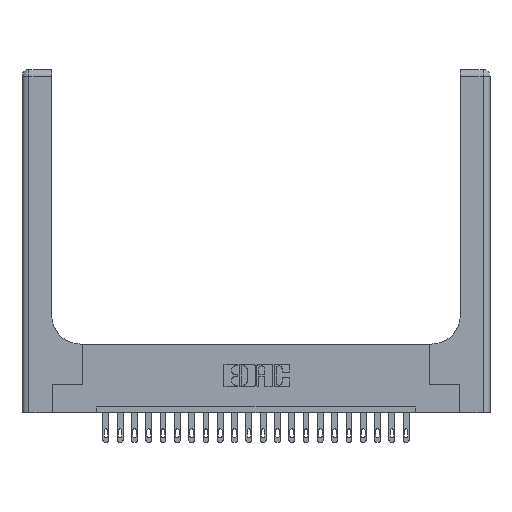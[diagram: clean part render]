
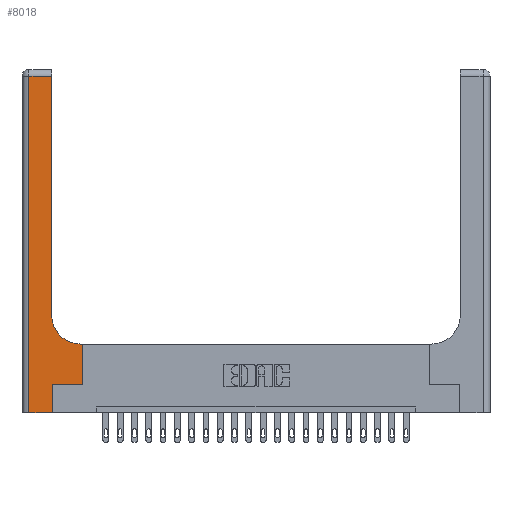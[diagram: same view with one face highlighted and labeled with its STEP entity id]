
A CAD part, top view. The second image highlights one B-rep face of the part: STEP entity #8018.
In plain terms, the highlighted planar face has unit normal (0, 0, 1).
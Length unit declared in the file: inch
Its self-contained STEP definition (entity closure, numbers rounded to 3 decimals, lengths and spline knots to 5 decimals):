
#81 = CARTESIAN_POINT ( 'NONE',  ( 0.528, 0.25, 0.37 ) ) ;
#326 = CARTESIAN_POINT ( 'NONE',  ( 0.26, 2.94, 0.37 ) ) ;
#426 = CARTESIAN_POINT ( 'NONE',  ( 0., 0., 0.37 ) ) ;
#790 = DIRECTION ( 'NONE',  ( 1., 0., 0. ) ) ;
#1011 = CARTESIAN_POINT ( 'NONE',  ( 0.265, 0., 0.37 ) ) ;
#1046 = DIRECTION ( 'NONE',  ( -1., 0., 0. ) ) ;
#1199 = DIRECTION ( 'NONE',  ( -1., 0., 0. ) ) ;
#1802 = CARTESIAN_POINT ( 'NONE',  ( 0.265, 0., 0.37 ) ) ;
#2324 = VERTEX_POINT ( 'NONE', #20525 ) ;
#2341 = CARTESIAN_POINT ( 'NONE',  ( 0.51, 0.85, 0.37 ) ) ;
#2616 = DIRECTION ( 'NONE',  ( 1., 0., 0. ) ) ;
#2735 = CIRCLE ( 'NONE', #18642, 0.25 ) ;
#2833 = VERTEX_POINT ( 'NONE', #18940 ) ;
#3242 = DIRECTION ( 'NONE',  ( 0., 1., 0. ) ) ;
#3520 = LINE ( 'NONE', #81, #6730 ) ;
#3695 = LINE ( 'NONE', #1802, #6019 ) ;
#4494 = CARTESIAN_POINT ( 'NONE',  ( 0., 2.94, 0.37 ) ) ;
#4508 = VECTOR ( 'NONE', #1046, 39.37008 ) ;
#5003 = EDGE_CURVE ( 'NONE', #10012, #18430, #2735, .T. ) ;
#5129 = ORIENTED_EDGE ( 'NONE', *, *, #12434, .T. ) ;
#5174 = DIRECTION ( 'NONE',  ( 0., 1., 0. ) ) ;
#5262 = VECTOR ( 'NONE', #20151, 39.37008 ) ;
#5644 = VERTEX_POINT ( 'NONE', #13246 ) ;
#5827 = DIRECTION ( 'NONE',  ( -1., 0., 0. ) ) ;
#5969 = EDGE_CURVE ( 'NONE', #21880, #2833, #12785, .T. ) ;
#6019 = VECTOR ( 'NONE', #3242, 39.37008 ) ;
#6056 = EDGE_CURVE ( 'NONE', #21258, #5644, #11017, .T. ) ;
#6388 = CARTESIAN_POINT ( 'NONE',  ( 0., 3., 0.37 ) ) ;
#6585 = CARTESIAN_POINT ( 'NONE',  ( 0.26, 0.85, 0.37 ) ) ;
#6639 = CARTESIAN_POINT ( 'NONE',  ( 0.26, 3., 0.37 ) ) ;
#6648 = ORIENTED_EDGE ( 'NONE', *, *, #17637, .T. ) ;
#6730 = VECTOR ( 'NONE', #5174, 39.37008 ) ;
#6843 = AXIS2_PLACEMENT_3D ( 'NONE', #6388, #21678, #1199 ) ;
#6996 = EDGE_CURVE ( 'NONE', #5644, #2324, #3520, .T. ) ;
#7869 = VECTOR ( 'NONE', #11109, 39.37008 ) ;
#7893 = EDGE_LOOP ( 'NONE', ( #6648, #17546, #5129, #21319, #10302, #15161, #16015, #21502, #9276 ) ) ;
#8018 = ADVANCED_FACE ( 'NONE', ( #15122 ), #19900, .F. ) ;
#9131 = EDGE_CURVE ( 'NONE', #10638, #21258, #3695, .T. ) ;
#9276 = ORIENTED_EDGE ( 'NONE', *, *, #5003, .T. ) ;
#10012 = VERTEX_POINT ( 'NONE', #17739 ) ;
#10067 = LINE ( 'NONE', #6639, #5262 ) ;
#10302 = ORIENTED_EDGE ( 'NONE', *, *, #9131, .T. ) ;
#10428 = VECTOR ( 'NONE', #13925, 39.37008 ) ;
#10638 = VERTEX_POINT ( 'NONE', #1011 ) ;
#10920 = EDGE_CURVE ( 'NONE', #21143, #10638, #15582, .T. ) ;
#11005 = CARTESIAN_POINT ( 'NONE',  ( 0.06, 3., 0.37 ) ) ;
#11017 = LINE ( 'NONE', #17767, #19483 ) ;
#11109 = DIRECTION ( 'NONE',  ( 0., -1., 0. ) ) ;
#12434 = EDGE_CURVE ( 'NONE', #2833, #21143, #19320, .T. ) ;
#12785 = LINE ( 'NONE', #4494, #20194 ) ;
#13246 = CARTESIAN_POINT ( 'NONE',  ( 0.528, 0.25, 0.37 ) ) ;
#13925 = DIRECTION ( 'NONE',  ( 1., 0., 0. ) ) ;
#15122 = FACE_OUTER_BOUND ( 'NONE', #7893, .T. ) ;
#15161 = ORIENTED_EDGE ( 'NONE', *, *, #6056, .T. ) ;
#15582 = LINE ( 'NONE', #426, #10428 ) ;
#15941 = DIRECTION ( 'NONE',  ( 0., 0., -1. ) ) ;
#16015 = ORIENTED_EDGE ( 'NONE', *, *, #6996, .T. ) ;
#16198 = LINE ( 'NONE', #19436, #4508 ) ;
#16996 = CARTESIAN_POINT ( 'NONE',  ( 0.06, 0., 0.37 ) ) ;
#17546 = ORIENTED_EDGE ( 'NONE', *, *, #5969, .T. ) ;
#17637 = EDGE_CURVE ( 'NONE', #18430, #21880, #10067, .T. ) ;
#17739 = CARTESIAN_POINT ( 'NONE',  ( 0.51, 0.6, 0.37 ) ) ;
#17767 = CARTESIAN_POINT ( 'NONE',  ( 0.265, 0.25, 0.37 ) ) ;
#17856 = CARTESIAN_POINT ( 'NONE',  ( 0.265, 0.25, 0.37 ) ) ;
#18430 = VERTEX_POINT ( 'NONE', #6585 ) ;
#18642 = AXIS2_PLACEMENT_3D ( 'NONE', #2341, #15941, #790 ) ;
#18940 = CARTESIAN_POINT ( 'NONE',  ( 0.06, 2.94, 0.37 ) ) ;
#19320 = LINE ( 'NONE', #11005, #7869 ) ;
#19436 = CARTESIAN_POINT ( 'NONE',  ( 0.26, 0.6, 0.37 ) ) ;
#19483 = VECTOR ( 'NONE', #2616, 39.37008 ) ;
#19900 = PLANE ( 'NONE',  #6843 ) ;
#20151 = DIRECTION ( 'NONE',  ( 0., 1., 0. ) ) ;
#20194 = VECTOR ( 'NONE', #5827, 39.37008 ) ;
#20525 = CARTESIAN_POINT ( 'NONE',  ( 0.528, 0.6, 0.37 ) ) ;
#21143 = VERTEX_POINT ( 'NONE', #16996 ) ;
#21173 = EDGE_CURVE ( 'NONE', #2324, #10012, #16198, .T. ) ;
#21258 = VERTEX_POINT ( 'NONE', #17856 ) ;
#21319 = ORIENTED_EDGE ( 'NONE', *, *, #10920, .T. ) ;
#21502 = ORIENTED_EDGE ( 'NONE', *, *, #21173, .T. ) ;
#21678 = DIRECTION ( 'NONE',  ( 0., 0., -1. ) ) ;
#21880 = VERTEX_POINT ( 'NONE', #326 ) ;
